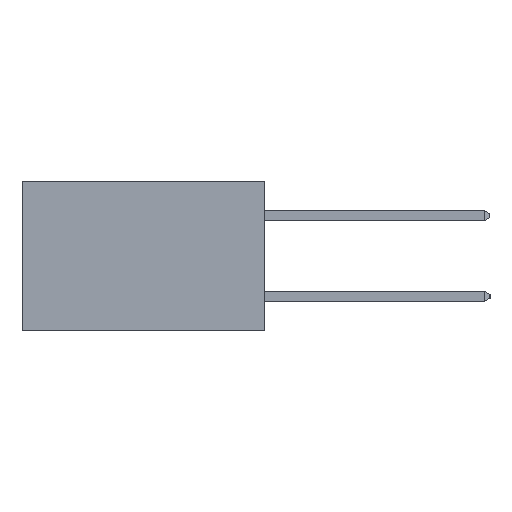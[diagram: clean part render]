
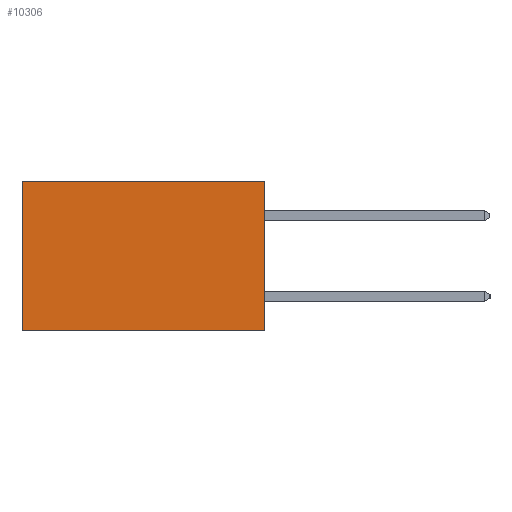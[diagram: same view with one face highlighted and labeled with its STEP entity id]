
A CAD part, left-side view. The second image highlights one B-rep face of the part: STEP entity #10306.
In plain terms, the highlighted planar face has unit normal (-1, 0, 0).
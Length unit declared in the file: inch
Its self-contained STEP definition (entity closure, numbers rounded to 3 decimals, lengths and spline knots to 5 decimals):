
#746 = VECTOR ( 'NONE', #1096, 39.37008 ) ;
#1096 = DIRECTION ( 'NONE',  ( 0., 0., -1. ) ) ;
#1100 = DIRECTION ( 'NONE',  ( 0., 1., 0. ) ) ;
#1217 = DIRECTION ( 'NONE',  ( 0., 0., -1. ) ) ;
#1806 = PLANE ( 'NONE',  #9414 ) ;
#2233 = EDGE_CURVE ( 'NONE', #16519, #4963, #8167, .T. ) ;
#2614 = VECTOR ( 'NONE', #10897, 39.37008 ) ;
#2621 = CARTESIAN_POINT ( 'NONE',  ( 0.2615, 0., 0. ) ) ;
#2968 = CARTESIAN_POINT ( 'NONE',  ( 0.2615, 0., -0.37 ) ) ;
#3328 = DIRECTION ( 'NONE',  ( 1., 0., 0. ) ) ;
#4136 = EDGE_CURVE ( 'NONE', #16519, #14329, #14086, .T. ) ;
#4963 = VERTEX_POINT ( 'NONE', #2968 ) ;
#5934 = EDGE_CURVE ( 'NONE', #4963, #14294, #13442, .T. ) ;
#6562 = LINE ( 'NONE', #11540, #17994 ) ;
#7553 = FACE_OUTER_BOUND ( 'NONE', #10923, .T. ) ;
#7837 = ORIENTED_EDGE ( 'NONE', *, *, #4136, .T. ) ;
#8167 = LINE ( 'NONE', #15927, #746 ) ;
#9414 = AXIS2_PLACEMENT_3D ( 'NONE', #16488, #3328, #13612 ) ;
#9896 = ORIENTED_EDGE ( 'NONE', *, *, #2233, .F. ) ;
#10306 = ADVANCED_FACE ( 'NONE', ( #7553 ), #1806, .F. ) ;
#10897 = DIRECTION ( 'NONE',  ( 0., 1., 0. ) ) ;
#10923 = EDGE_LOOP ( 'NONE', ( #15792, #18431, #9896, #7837 ) ) ;
#11540 = CARTESIAN_POINT ( 'NONE',  ( 0.2615, 0.6, -0.37 ) ) ;
#11594 = CARTESIAN_POINT ( 'NONE',  ( 0.2615, 0.6, -0.37 ) ) ;
#13141 = CARTESIAN_POINT ( 'NONE',  ( 0.2615, 0.6, 0. ) ) ;
#13442 = LINE ( 'NONE', #18210, #2614 ) ;
#13612 = DIRECTION ( 'NONE',  ( 0., 0., -1. ) ) ;
#13616 = CARTESIAN_POINT ( 'NONE',  ( 0.2615, 0., 0. ) ) ;
#13862 = EDGE_CURVE ( 'NONE', #14329, #14294, #6562, .T. ) ;
#14086 = LINE ( 'NONE', #2621, #17501 ) ;
#14294 = VERTEX_POINT ( 'NONE', #11594 ) ;
#14329 = VERTEX_POINT ( 'NONE', #13141 ) ;
#15792 = ORIENTED_EDGE ( 'NONE', *, *, #13862, .T. ) ;
#15927 = CARTESIAN_POINT ( 'NONE',  ( 0.2615, 0., -0.37 ) ) ;
#16488 = CARTESIAN_POINT ( 'NONE',  ( 0.2615, 0., -0.37 ) ) ;
#16519 = VERTEX_POINT ( 'NONE', #13616 ) ;
#17501 = VECTOR ( 'NONE', #1100, 39.37008 ) ;
#17994 = VECTOR ( 'NONE', #1217, 39.37008 ) ;
#18210 = CARTESIAN_POINT ( 'NONE',  ( 0.2615, 0., -0.37 ) ) ;
#18431 = ORIENTED_EDGE ( 'NONE', *, *, #5934, .F. ) ;
